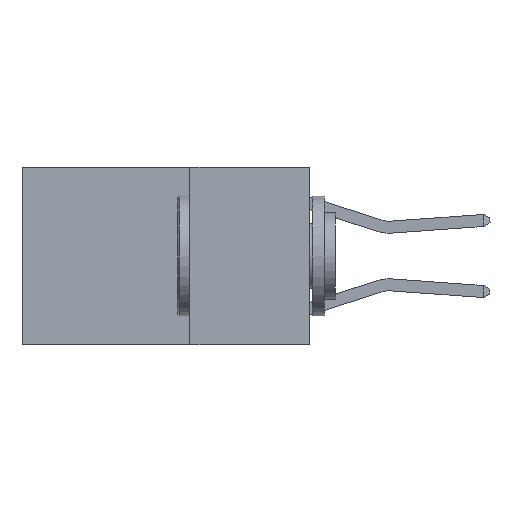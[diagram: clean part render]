
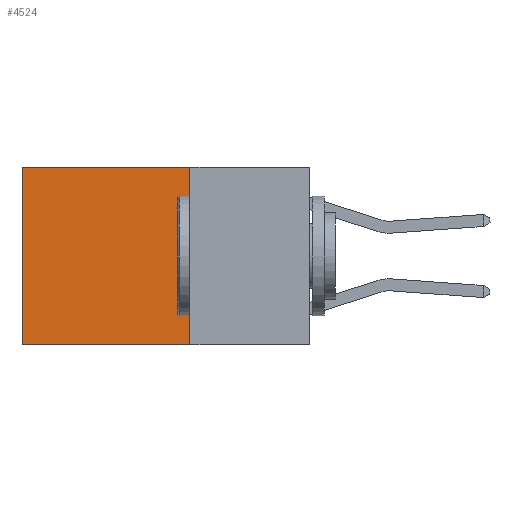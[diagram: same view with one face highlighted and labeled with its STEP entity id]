
A CAD part, left-side view. The second image highlights one B-rep face of the part: STEP entity #4524.
In plain terms, the highlighted planar face has unit normal (-1, 0, 0).
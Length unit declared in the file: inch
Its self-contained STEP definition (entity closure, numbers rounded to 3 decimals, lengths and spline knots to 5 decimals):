
#870 = PLANE ( 'NONE',  #5392 ) ;
#1221 = FACE_OUTER_BOUND ( 'NONE', #2073, .T. ) ;
#1830 = VERTEX_POINT ( 'NONE', #11197 ) ;
#2046 = DIRECTION ( 'NONE',  ( 0., 0., -1. ) ) ;
#2073 = EDGE_LOOP ( 'NONE', ( #9198, #7286, #11162, #10925 ) ) ;
#2077 = CARTESIAN_POINT ( 'NONE',  ( 0.2625, 0.6, 0. ) ) ;
#2591 = DIRECTION ( 'NONE',  ( 0., 1., 0. ) ) ;
#2596 = DIRECTION ( 'NONE',  ( 0., 0., -1. ) ) ;
#3582 = DIRECTION ( 'NONE',  ( 1., 0., 0. ) ) ;
#4227 = CARTESIAN_POINT ( 'NONE',  ( 0.2625, 0.25, 0. ) ) ;
#4312 = VECTOR ( 'NONE', #11244, 39.37008 ) ;
#4468 = EDGE_CURVE ( 'NONE', #9681, #11565, #11914, .T. ) ;
#4524 = ADVANCED_FACE ( 'NONE', ( #1221 ), #870, .F. ) ;
#4979 = VERTEX_POINT ( 'NONE', #2077 ) ;
#5392 = AXIS2_PLACEMENT_3D ( 'NONE', #7393, #3582, #2596 ) ;
#5429 = LINE ( 'NONE', #7307, #7507 ) ;
#6866 = VECTOR ( 'NONE', #2046, 39.37008 ) ;
#7245 = CARTESIAN_POINT ( 'NONE',  ( 0.2625, 0.25, -0.37 ) ) ;
#7286 = ORIENTED_EDGE ( 'NONE', *, *, #8177, .F. ) ;
#7307 = CARTESIAN_POINT ( 'NONE',  ( 0.2625, 0.25, -0.37 ) ) ;
#7393 = CARTESIAN_POINT ( 'NONE',  ( 0.2625, 0.25, 0. ) ) ;
#7507 = VECTOR ( 'NONE', #2591, 39.37008 ) ;
#7675 = CARTESIAN_POINT ( 'NONE',  ( 0.2625, 0.6, 0. ) ) ;
#8177 = EDGE_CURVE ( 'NONE', #11565, #1830, #5429, .T. ) ;
#8318 = DIRECTION ( 'NONE',  ( 0., 0., -1. ) ) ;
#9198 = ORIENTED_EDGE ( 'NONE', *, *, #11183, .T. ) ;
#9681 = VERTEX_POINT ( 'NONE', #4227 ) ;
#9984 = CARTESIAN_POINT ( 'NONE',  ( 0.2625, 0.25, 0. ) ) ;
#10393 = LINE ( 'NONE', #12062, #4312 ) ;
#10925 = ORIENTED_EDGE ( 'NONE', *, *, #11578, .T. ) ;
#11128 = LINE ( 'NONE', #7675, #6866 ) ;
#11162 = ORIENTED_EDGE ( 'NONE', *, *, #4468, .F. ) ;
#11183 = EDGE_CURVE ( 'NONE', #4979, #1830, #11128, .T. ) ;
#11197 = CARTESIAN_POINT ( 'NONE',  ( 0.2625, 0.6, -0.37 ) ) ;
#11199 = VECTOR ( 'NONE', #8318, 39.37008 ) ;
#11244 = DIRECTION ( 'NONE',  ( 0., 1., 0. ) ) ;
#11565 = VERTEX_POINT ( 'NONE', #7245 ) ;
#11578 = EDGE_CURVE ( 'NONE', #9681, #4979, #10393, .T. ) ;
#11914 = LINE ( 'NONE', #9984, #11199 ) ;
#12062 = CARTESIAN_POINT ( 'NONE',  ( 0.2625, 0.25, 0. ) ) ;
